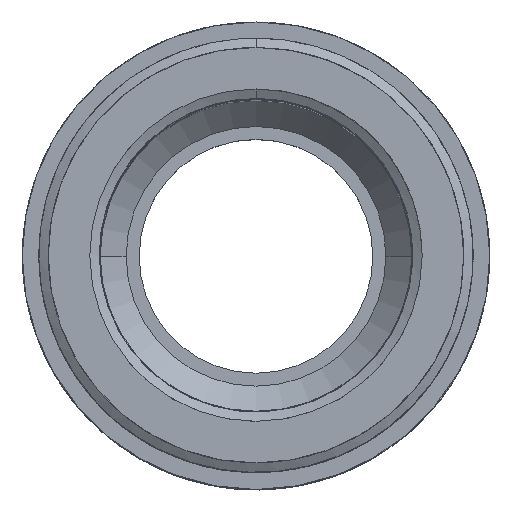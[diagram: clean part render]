
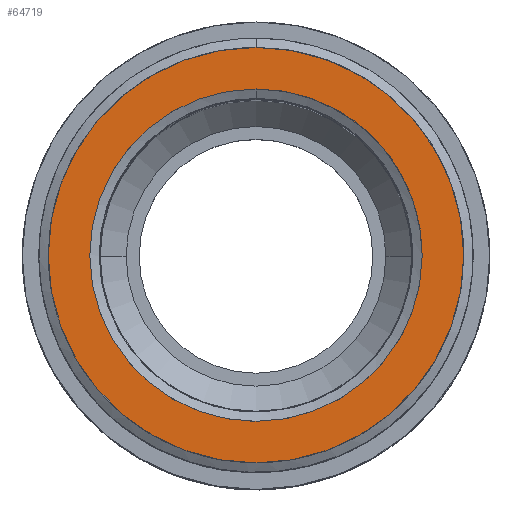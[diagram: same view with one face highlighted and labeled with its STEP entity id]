
A CAD part, top view. The second image highlights one B-rep face of the part: STEP entity #64719.
In plain terms, the highlighted planar face has unit normal (0, 0, 1).
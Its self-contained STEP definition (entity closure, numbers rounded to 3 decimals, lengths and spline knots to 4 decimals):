
#4639 = CARTESIAN_POINT ( 'NONE',  ( -0.8, 0., 3.5 ) ) ;
#7916 = DIRECTION ( 'NONE',  ( -1., 0., 0. ) ) ;
#8606 = DIRECTION ( 'NONE',  ( 1., 0., 0. ) ) ;
#8705 = ORIENTED_EDGE ( 'NONE', *, *, #62741, .T. ) ;
#10457 = EDGE_CURVE ( 'NONE', #44788, #70713, #43114, .T. ) ;
#12035 = DIRECTION ( 'NONE',  ( 0., 0., 1. ) ) ;
#16948 = ORIENTED_EDGE ( 'NONE', *, *, #36657, .T. ) ;
#17889 = FACE_OUTER_BOUND ( 'NONE', #64748, .T. ) ;
#19616 = VERTEX_POINT ( 'NONE', #41699 ) ;
#20809 = DIRECTION ( 'NONE',  ( 1., 0., 0. ) ) ;
#22190 = DIRECTION ( 'NONE',  ( 0., 0., -1. ) ) ;
#24732 = CARTESIAN_POINT ( 'NONE',  ( 0.8, 0., 3.5 ) ) ;
#24838 = EDGE_LOOP ( 'NONE', ( #67940, #81225, #16948 ) ) ;
#26551 = DIRECTION ( 'NONE',  ( 0., 0., -1. ) ) ;
#31802 = CIRCLE ( 'NONE', #102113, 0.8 ) ;
#32432 = VERTEX_POINT ( 'NONE', #24732 ) ;
#32895 = CARTESIAN_POINT ( 'NONE',  ( 0., 0., 3.5 ) ) ;
#33002 = VERTEX_POINT ( 'NONE', #103565 ) ;
#34429 = ORIENTED_EDGE ( 'NONE', *, *, #48391, .T. ) ;
#36657 = EDGE_CURVE ( 'NONE', #56450, #33002, #69293, .T. ) ;
#38040 = CIRCLE ( 'NONE', #42751, 1. ) ;
#38067 = CARTESIAN_POINT ( 'NONE',  ( 0., 0., 3.5 ) ) ;
#41479 = CIRCLE ( 'NONE', #90674, 0.8 ) ;
#41699 = CARTESIAN_POINT ( 'NONE',  ( 1., 0., 3.5 ) ) ;
#42751 = AXIS2_PLACEMENT_3D ( 'NONE', #54989, #79911, #47201 ) ;
#43114 = CIRCLE ( 'NONE', #97344, 1. ) ;
#43127 = AXIS2_PLACEMENT_3D ( 'NONE', #77130, #12035, #60646 ) ;
#44788 = VERTEX_POINT ( 'NONE', #86407 ) ;
#46476 = DIRECTION ( 'NONE',  ( -1., 0., 0. ) ) ;
#47201 = DIRECTION ( 'NONE',  ( 1., 0., 0. ) ) ;
#48391 = EDGE_CURVE ( 'NONE', #19616, #44788, #68082, .T. ) ;
#50123 = DIRECTION ( 'NONE',  ( -1., 0., 0. ) ) ;
#53201 = CARTESIAN_POINT ( 'NONE',  ( 0., 0., 3.5 ) ) ;
#54989 = CARTESIAN_POINT ( 'NONE',  ( 0., 0., 3.5 ) ) ;
#56450 = VERTEX_POINT ( 'NONE', #4639 ) ;
#58957 = CARTESIAN_POINT ( 'NONE',  ( 0., 0., 3.5 ) ) ;
#60646 = DIRECTION ( 'NONE',  ( 1., 0., 0. ) ) ;
#62741 = EDGE_CURVE ( 'NONE', #70713, #19616, #38040, .T. ) ;
#64719 = ADVANCED_FACE ( 'NONE', ( #100955, #17889 ), #89183, .T. ) ;
#64748 = EDGE_LOOP ( 'NONE', ( #69521, #8705, #34429 ) ) ;
#67940 = ORIENTED_EDGE ( 'NONE', *, *, #93675, .T. ) ;
#68082 = CIRCLE ( 'NONE', #43127, 1. ) ;
#69293 = CIRCLE ( 'NONE', #92538, 0.8 ) ;
#69521 = ORIENTED_EDGE ( 'NONE', *, *, #10457, .T. ) ;
#69847 = AXIS2_PLACEMENT_3D ( 'NONE', #32895, #96862, #8606 ) ;
#70586 = EDGE_CURVE ( 'NONE', #32432, #56450, #41479, .T. ) ;
#70713 = VERTEX_POINT ( 'NONE', #75473 ) ;
#75473 = CARTESIAN_POINT ( 'NONE',  ( -1., 0., 3.5 ) ) ;
#77130 = CARTESIAN_POINT ( 'NONE',  ( 0., 0., 3.5 ) ) ;
#79911 = DIRECTION ( 'NONE',  ( 0., 0., 1. ) ) ;
#81225 = ORIENTED_EDGE ( 'NONE', *, *, #70586, .T. ) ;
#86407 = CARTESIAN_POINT ( 'NONE',  ( 0., 1., 3.5 ) ) ;
#88141 = DIRECTION ( 'NONE',  ( 0., 0., -1. ) ) ;
#89183 = PLANE ( 'NONE',  #69847 ) ;
#90674 = AXIS2_PLACEMENT_3D ( 'NONE', #58957, #26551, #50123 ) ;
#92538 = AXIS2_PLACEMENT_3D ( 'NONE', #53201, #22190, #46476 ) ;
#93675 = EDGE_CURVE ( 'NONE', #33002, #32432, #31802, .T. ) ;
#94308 = DIRECTION ( 'NONE',  ( 0., 0., 1. ) ) ;
#96862 = DIRECTION ( 'NONE',  ( 0., 0., 1. ) ) ;
#97344 = AXIS2_PLACEMENT_3D ( 'NONE', #38067, #94308, #20809 ) ;
#100955 = FACE_BOUND ( 'NONE', #24838, .T. ) ;
#102113 = AXIS2_PLACEMENT_3D ( 'NONE', #103554, #88141, #7916 ) ;
#103554 = CARTESIAN_POINT ( 'NONE',  ( 0., 0., 3.5 ) ) ;
#103565 = CARTESIAN_POINT ( 'NONE',  ( 0., 0.8, 3.5 ) ) ;
